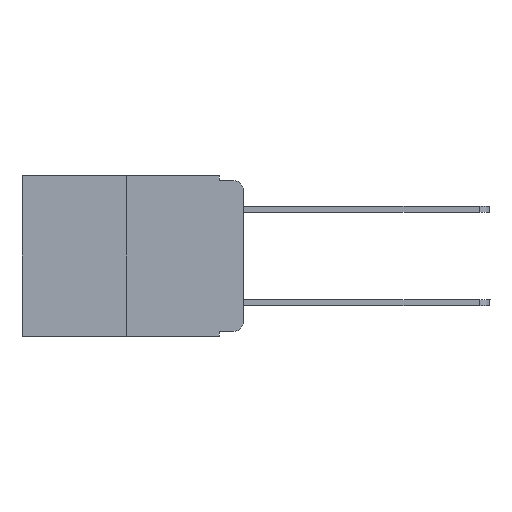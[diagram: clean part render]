
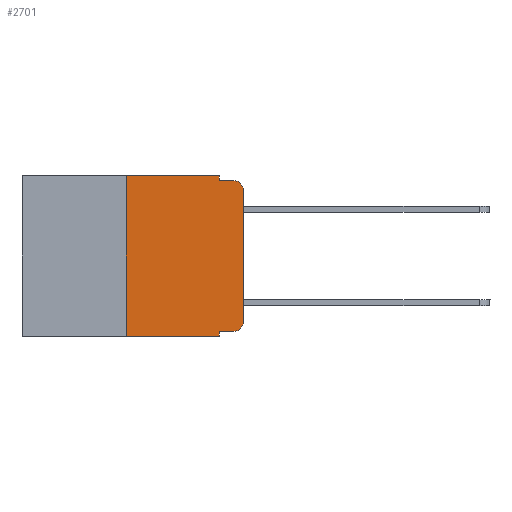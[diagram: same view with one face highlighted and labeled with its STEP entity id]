
A CAD part, left-side view. The second image highlights one B-rep face of the part: STEP entity #2701.
In plain terms, the highlighted planar face has unit normal (-1, 0, 0).
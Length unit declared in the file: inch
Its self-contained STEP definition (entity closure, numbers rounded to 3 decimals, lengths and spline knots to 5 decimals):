
#62 = AXIS2_PLACEMENT_3D ( 'NONE', #906, #13842, #11416 ) ;
#127 = FACE_OUTER_BOUND ( 'NONE', #2476, .T. ) ;
#179 = VECTOR ( 'NONE', #16054, 39.37008 ) ;
#495 = LINE ( 'NONE', #1621, #5368 ) ;
#663 = DIRECTION ( 'NONE',  ( 0., 0., -1. ) ) ;
#906 = CARTESIAN_POINT ( 'NONE',  ( 0., 0.02, -0.313 ) ) ;
#944 = CARTESIAN_POINT ( 'NONE',  ( 0., 0.25, -0.343 ) ) ;
#1370 = DIRECTION ( 'NONE',  ( 0., 0., -1. ) ) ;
#1458 = LINE ( 'NONE', #2842, #12073 ) ;
#1495 = VERTEX_POINT ( 'NONE', #15591 ) ;
#1621 = CARTESIAN_POINT ( 'NONE',  ( 0., 0.473, 0. ) ) ;
#1865 = ORIENTED_EDGE ( 'NONE', *, *, #2383, .F. ) ;
#1893 = LINE ( 'NONE', #5512, #179 ) ;
#2002 = VECTOR ( 'NONE', #10531, 39.37008 ) ;
#2383 = EDGE_CURVE ( 'NONE', #7511, #11687, #495, .T. ) ;
#2476 = EDGE_LOOP ( 'NONE', ( #2746, #15102, #3135, #8282, #1865, #6134, #2934, #11452, #8615, #11650 ) ) ;
#2557 = DIRECTION ( 'NONE',  ( 0., 0., -1. ) ) ;
#2660 = CARTESIAN_POINT ( 'NONE',  ( 0., 0.051, -0.01 ) ) ;
#2701 = ADVANCED_FACE ( 'NONE', ( #127 ), #10471, .F. ) ;
#2723 = CARTESIAN_POINT ( 'NONE',  ( 0., 0.473, 0. ) ) ;
#2733 = CARTESIAN_POINT ( 'NONE',  ( 0., 0.051, 0. ) ) ;
#2746 = ORIENTED_EDGE ( 'NONE', *, *, #16408, .T. ) ;
#2842 = CARTESIAN_POINT ( 'NONE',  ( 0., 0.051, 0. ) ) ;
#2934 = ORIENTED_EDGE ( 'NONE', *, *, #4151, .T. ) ;
#2960 = EDGE_CURVE ( 'NONE', #4814, #7545, #16627, .T. ) ;
#3002 = LINE ( 'NONE', #6525, #13896 ) ;
#3135 = ORIENTED_EDGE ( 'NONE', *, *, #16945, .F. ) ;
#3141 = VERTEX_POINT ( 'NONE', #5284 ) ;
#3812 = LINE ( 'NONE', #6473, #9956 ) ;
#4073 = AXIS2_PLACEMENT_3D ( 'NONE', #14020, #15328, #663 ) ;
#4151 = EDGE_CURVE ( 'NONE', #15648, #10334, #3002, .T. ) ;
#4690 = LINE ( 'NONE', #11324, #2002 ) ;
#4814 = VERTEX_POINT ( 'NONE', #8760 ) ;
#4887 = EDGE_CURVE ( 'NONE', #1495, #4814, #4690, .T. ) ;
#5284 = CARTESIAN_POINT ( 'NONE',  ( 0., 0., -0.03 ) ) ;
#5368 = VECTOR ( 'NONE', #13524, 39.37008 ) ;
#5401 = LINE ( 'NONE', #2733, #9581 ) ;
#5512 = CARTESIAN_POINT ( 'NONE',  ( 0., 0.25, 0. ) ) ;
#6134 = ORIENTED_EDGE ( 'NONE', *, *, #7228, .F. ) ;
#6473 = CARTESIAN_POINT ( 'NONE',  ( 0., 0., 0. ) ) ;
#6525 = CARTESIAN_POINT ( 'NONE',  ( 0., 0.473, -0.343 ) ) ;
#6554 = DIRECTION ( 'NONE',  ( 0., 0., 1. ) ) ;
#6579 = CARTESIAN_POINT ( 'NONE',  ( 0., 0.051, 0. ) ) ;
#7228 = EDGE_CURVE ( 'NONE', #15648, #7511, #1893, .T. ) ;
#7511 = VERTEX_POINT ( 'NONE', #16551 ) ;
#7545 = VERTEX_POINT ( 'NONE', #11156 ) ;
#8282 = ORIENTED_EDGE ( 'NONE', *, *, #12055, .F. ) ;
#8615 = ORIENTED_EDGE ( 'NONE', *, *, #4887, .T. ) ;
#8760 = CARTESIAN_POINT ( 'NONE',  ( 0., 0.02, -0.333 ) ) ;
#8893 = VECTOR ( 'NONE', #15967, 39.37008 ) ;
#9567 = VERTEX_POINT ( 'NONE', #15455 ) ;
#9581 = VECTOR ( 'NONE', #2557, 39.37008 ) ;
#9956 = VECTOR ( 'NONE', #6554, 39.37008 ) ;
#10113 = EDGE_CURVE ( 'NONE', #1495, #10334, #5401, .T. ) ;
#10334 = VERTEX_POINT ( 'NONE', #14105 ) ;
#10471 = PLANE ( 'NONE',  #13846 ) ;
#10531 = DIRECTION ( 'NONE',  ( 0., -1., 0. ) ) ;
#11059 = VERTEX_POINT ( 'NONE', #16850 ) ;
#11156 = CARTESIAN_POINT ( 'NONE',  ( 0., 0., -0.313 ) ) ;
#11324 = CARTESIAN_POINT ( 'NONE',  ( 0., 0.051, -0.333 ) ) ;
#11416 = DIRECTION ( 'NONE',  ( 0., 0., -1. ) ) ;
#11452 = ORIENTED_EDGE ( 'NONE', *, *, #10113, .F. ) ;
#11650 = ORIENTED_EDGE ( 'NONE', *, *, #2960, .T. ) ;
#11687 = VERTEX_POINT ( 'NONE', #6579 ) ;
#12055 = EDGE_CURVE ( 'NONE', #11687, #11059, #1458, .T. ) ;
#12073 = VECTOR ( 'NONE', #1370, 39.37008 ) ;
#12817 = EDGE_CURVE ( 'NONE', #3141, #9567, #13989, .T. ) ;
#13226 = DIRECTION ( 'NONE',  ( 0., 0., -1. ) ) ;
#13245 = DIRECTION ( 'NONE',  ( 0., -1., 0. ) ) ;
#13524 = DIRECTION ( 'NONE',  ( 0., -1., 0. ) ) ;
#13842 = DIRECTION ( 'NONE',  ( -1., 0., 0. ) ) ;
#13846 = AXIS2_PLACEMENT_3D ( 'NONE', #2723, #15762, #13226 ) ;
#13896 = VECTOR ( 'NONE', #13245, 39.37008 ) ;
#13989 = CIRCLE ( 'NONE', #4073, 0.02 ) ;
#14020 = CARTESIAN_POINT ( 'NONE',  ( 0., 0.02, -0.03 ) ) ;
#14105 = CARTESIAN_POINT ( 'NONE',  ( 0., 0.051, -0.343 ) ) ;
#15102 = ORIENTED_EDGE ( 'NONE', *, *, #12817, .T. ) ;
#15328 = DIRECTION ( 'NONE',  ( -1., 0., 0. ) ) ;
#15455 = CARTESIAN_POINT ( 'NONE',  ( 0., 0.02, -0.01 ) ) ;
#15591 = CARTESIAN_POINT ( 'NONE',  ( 0., 0.051, -0.333 ) ) ;
#15648 = VERTEX_POINT ( 'NONE', #944 ) ;
#15762 = DIRECTION ( 'NONE',  ( 1., 0., 0. ) ) ;
#15873 = LINE ( 'NONE', #2660, #8893 ) ;
#15967 = DIRECTION ( 'NONE',  ( 0., -1., 0. ) ) ;
#16054 = DIRECTION ( 'NONE',  ( 0., 0., 1. ) ) ;
#16408 = EDGE_CURVE ( 'NONE', #7545, #3141, #3812, .T. ) ;
#16551 = CARTESIAN_POINT ( 'NONE',  ( 0., 0.25, 0. ) ) ;
#16627 = CIRCLE ( 'NONE', #62, 0.02 ) ;
#16850 = CARTESIAN_POINT ( 'NONE',  ( 0., 0.051, -0.01 ) ) ;
#16945 = EDGE_CURVE ( 'NONE', #11059, #9567, #15873, .T. ) ;
